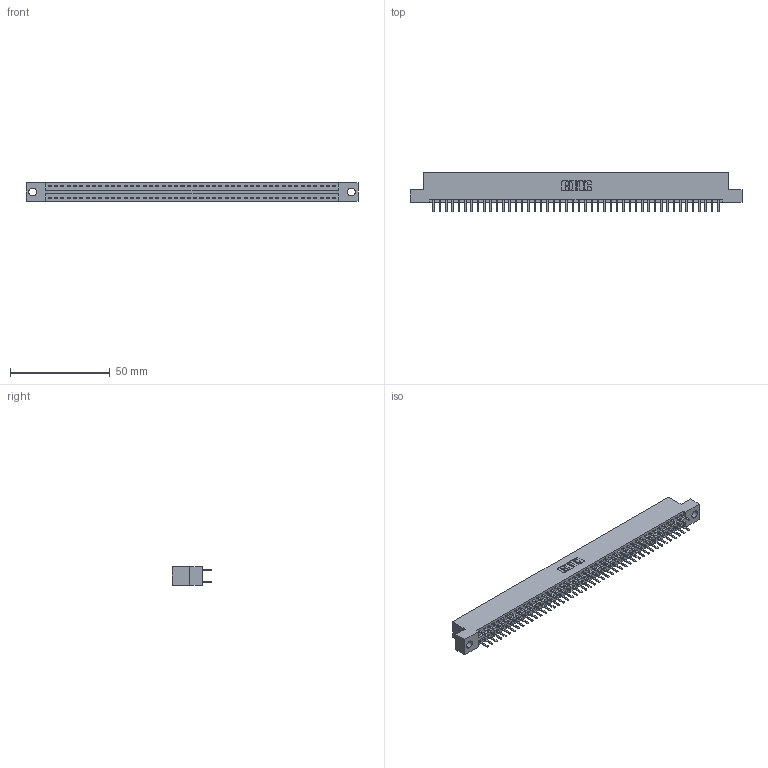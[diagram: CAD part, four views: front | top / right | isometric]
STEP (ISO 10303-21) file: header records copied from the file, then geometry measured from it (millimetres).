
FILE_DESCRIPTION (( 'STEP AP203' ), '1' );
FILE_NAME ('346-092-520-204.STEP', '2022-05-26T06:03:54', ( '' ), ( '' ), 'SwSTEP 2.0', 'SolidWorks 2020', '' );
FILE_SCHEMA (( 'CONFIG_CONTROL_DESIGN' ));
Length unit declared in the file: inch
Products named in the file (3): 345-292-001_345-293-120; 346 Part_Flush Mounting Lugs - 0.156 Dia-TH; 346-092-520-204
Assembly tree (93 placements, depth 2):
  346-092-520-204
    346 Part_Flush Mounting Lugs - 0.156 Dia-TH
    345-292-001_345-293-120  x92
Bounding box: 166.62 x 20.02 x 9.4 mm (x, y, z)
Volume: 16132.6 mm3; surface area: 21991.3 mm2
Topology: 93 solids, 93 shells, 5288 faces, 15361 edges, 9994 vertices
Faces by surface type: plane 3494, cylinder 1794
Entity records: 30015 total; most frequent: CARTESIAN_POINT 4958, ORIENTED_EDGE 4878, DIRECTION 4407, EDGE_CURVE 2439, VECTOR 2119, LINE 2119, VERTEX_POINT 1622, AXIS2_PLACEMENT_3D 1144
